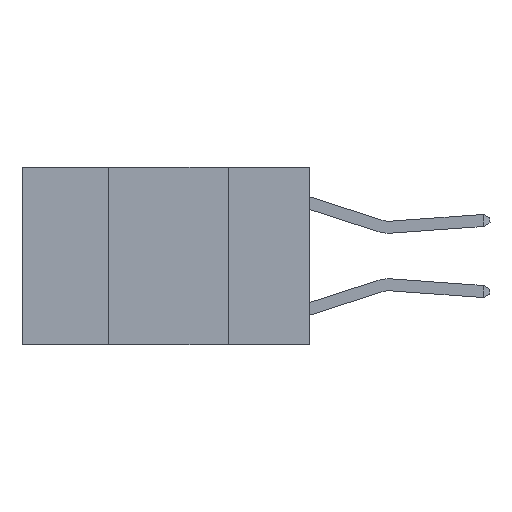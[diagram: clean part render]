
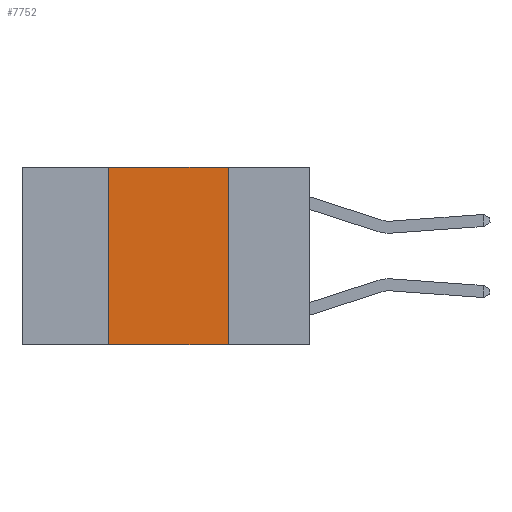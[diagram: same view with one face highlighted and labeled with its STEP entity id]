
A CAD part, left-side view. The second image highlights one B-rep face of the part: STEP entity #7752.
In plain terms, the highlighted planar face has unit normal (-1, 0, 0).
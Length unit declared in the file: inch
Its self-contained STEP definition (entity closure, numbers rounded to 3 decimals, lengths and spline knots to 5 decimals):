
#82 = PLANE ( 'NONE',  #6228 ) ;
#305 = VECTOR ( 'NONE', #2917, 39.37008 ) ;
#650 = CARTESIAN_POINT ( 'NONE',  ( 0., 0.17, 0. ) ) ;
#731 = DIRECTION ( 'NONE',  ( 0., 0., -1. ) ) ;
#1326 = VECTOR ( 'NONE', #7066, 39.37008 ) ;
#1526 = LINE ( 'NONE', #5158, #1326 ) ;
#2858 = EDGE_CURVE ( 'NONE', #8120, #6301, #1526, .T. ) ;
#2917 = DIRECTION ( 'NONE',  ( 0., 0., 1. ) ) ;
#3026 = ORIENTED_EDGE ( 'NONE', *, *, #2858, .F. ) ;
#3308 = EDGE_CURVE ( 'NONE', #5603, #8287, #7504, .T. ) ;
#3455 = ORIENTED_EDGE ( 'NONE', *, *, #3308, .T. ) ;
#3505 = CARTESIAN_POINT ( 'NONE',  ( 0., 0.17, 0. ) ) ;
#3592 = CARTESIAN_POINT ( 'NONE',  ( 0., 0.42, 0. ) ) ;
#3836 = LINE ( 'NONE', #650, #6888 ) ;
#4294 = EDGE_LOOP ( 'NONE', ( #6332, #3026, #6728, #3455 ) ) ;
#4513 = DIRECTION ( 'NONE',  ( 0., -1., 0. ) ) ;
#5158 = CARTESIAN_POINT ( 'NONE',  ( 0., 0.6, 0. ) ) ;
#5570 = EDGE_CURVE ( 'NONE', #5603, #8120, #7521, .T. ) ;
#5603 = VERTEX_POINT ( 'NONE', #5632 ) ;
#5632 = CARTESIAN_POINT ( 'NONE',  ( 0., 0.42, -0.37 ) ) ;
#6228 = AXIS2_PLACEMENT_3D ( 'NONE', #7964, #6683, #731 ) ;
#6301 = VERTEX_POINT ( 'NONE', #3505 ) ;
#6332 = ORIENTED_EDGE ( 'NONE', *, *, #7676, .F. ) ;
#6490 = FACE_OUTER_BOUND ( 'NONE', #4294, .T. ) ;
#6605 = DIRECTION ( 'NONE',  ( 0., 0., -1. ) ) ;
#6683 = DIRECTION ( 'NONE',  ( 1., 0., 0. ) ) ;
#6728 = ORIENTED_EDGE ( 'NONE', *, *, #5570, .F. ) ;
#6888 = VECTOR ( 'NONE', #6605, 39.37008 ) ;
#7066 = DIRECTION ( 'NONE',  ( 0., -1., 0. ) ) ;
#7180 = CARTESIAN_POINT ( 'NONE',  ( 0., 0.42, 0. ) ) ;
#7504 = LINE ( 'NONE', #7681, #7707 ) ;
#7521 = LINE ( 'NONE', #3592, #305 ) ;
#7676 = EDGE_CURVE ( 'NONE', #6301, #8287, #3836, .T. ) ;
#7681 = CARTESIAN_POINT ( 'NONE',  ( 0., 0.6, -0.37 ) ) ;
#7707 = VECTOR ( 'NONE', #4513, 39.37008 ) ;
#7752 = ADVANCED_FACE ( 'NONE', ( #6490 ), #82, .F. ) ;
#7964 = CARTESIAN_POINT ( 'NONE',  ( 0., 0.6, 0. ) ) ;
#7989 = CARTESIAN_POINT ( 'NONE',  ( 0., 0.17, -0.37 ) ) ;
#8120 = VERTEX_POINT ( 'NONE', #7180 ) ;
#8287 = VERTEX_POINT ( 'NONE', #7989 ) ;
